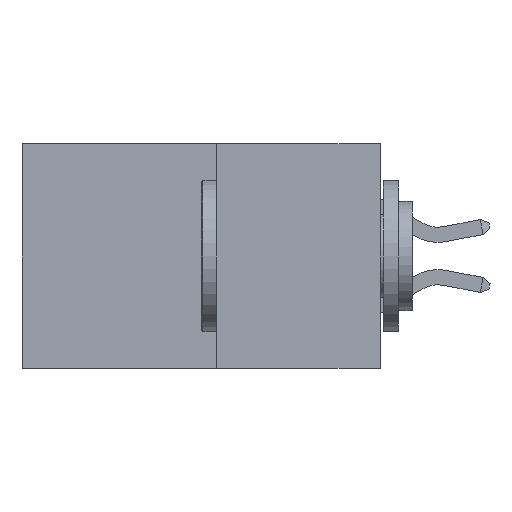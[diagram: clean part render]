
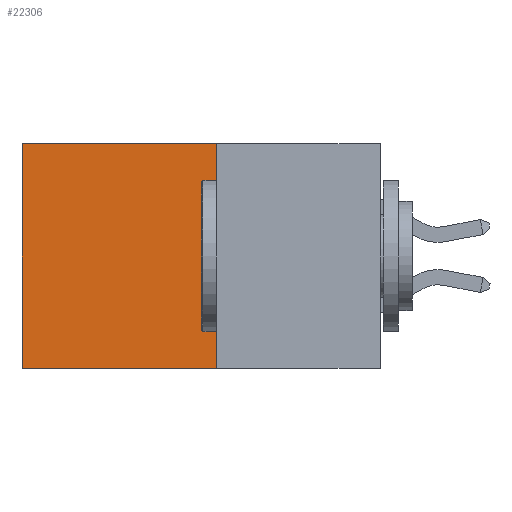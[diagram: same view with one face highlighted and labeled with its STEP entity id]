
A CAD part, left-side view. The second image highlights one B-rep face of the part: STEP entity #22306.
In plain terms, the highlighted planar face has unit normal (-1, 0, 0).
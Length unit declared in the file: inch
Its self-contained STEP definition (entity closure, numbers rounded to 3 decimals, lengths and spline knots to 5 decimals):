
#180 = ORIENTED_EDGE ( 'NONE', *, *, #5512, .T. ) ;
#1679 = AXIS2_PLACEMENT_3D ( 'NONE', #9399, #27180, #11938 ) ;
#3435 = CARTESIAN_POINT ( 'NONE',  ( 0.277, 0.27, 0. ) ) ;
#4235 = PLANE ( 'NONE',  #1679 ) ;
#5512 = EDGE_CURVE ( 'NONE', #9142, #13987, #30243, .T. ) ;
#5621 = EDGE_CURVE ( 'NONE', #30996, #9142, #13556, .T. ) ;
#6481 = CARTESIAN_POINT ( 'NONE',  ( 0.277, 0.59, -0.37 ) ) ;
#7763 = DIRECTION ( 'NONE',  ( 0., 0., -1. ) ) ;
#8308 = DIRECTION ( 'NONE',  ( 0., 1., 0. ) ) ;
#9009 = VECTOR ( 'NONE', #21920, 39.37008 ) ;
#9142 = VERTEX_POINT ( 'NONE', #32840 ) ;
#9253 = FACE_OUTER_BOUND ( 'NONE', #22468, .T. ) ;
#9399 = CARTESIAN_POINT ( 'NONE',  ( 0.277, 0.27, -0.37 ) ) ;
#11687 = CARTESIAN_POINT ( 'NONE',  ( 0.277, 0.27, -0.37 ) ) ;
#11938 = DIRECTION ( 'NONE',  ( 0., 0., -1. ) ) ;
#12021 = VERTEX_POINT ( 'NONE', #28474 ) ;
#12322 = EDGE_CURVE ( 'NONE', #12021, #13987, #23299, .T. ) ;
#13023 = ORIENTED_EDGE ( 'NONE', *, *, #12322, .F. ) ;
#13556 = LINE ( 'NONE', #21056, #19502 ) ;
#13987 = VERTEX_POINT ( 'NONE', #29155 ) ;
#14317 = ORIENTED_EDGE ( 'NONE', *, *, #27354, .F. ) ;
#17378 = VECTOR ( 'NONE', #19501, 39.37008 ) ;
#17708 = ORIENTED_EDGE ( 'NONE', *, *, #5621, .T. ) ;
#19501 = DIRECTION ( 'NONE',  ( 0., 0., -1. ) ) ;
#19502 = VECTOR ( 'NONE', #8308, 39.37008 ) ;
#21056 = CARTESIAN_POINT ( 'NONE',  ( 0.277, 0.27, 0. ) ) ;
#21920 = DIRECTION ( 'NONE',  ( 0., 1., 0. ) ) ;
#22306 = ADVANCED_FACE ( 'NONE', ( #9253 ), #4235, .F. ) ;
#22468 = EDGE_LOOP ( 'NONE', ( #180, #13023, #14317, #17708 ) ) ;
#23299 = LINE ( 'NONE', #11687, #9009 ) ;
#23492 = VECTOR ( 'NONE', #7763, 39.37008 ) ;
#27180 = DIRECTION ( 'NONE',  ( 1., 0., 0. ) ) ;
#27354 = EDGE_CURVE ( 'NONE', #30996, #12021, #31601, .T. ) ;
#28474 = CARTESIAN_POINT ( 'NONE',  ( 0.277, 0.27, -0.37 ) ) ;
#29155 = CARTESIAN_POINT ( 'NONE',  ( 0.277, 0.59, -0.37 ) ) ;
#29611 = CARTESIAN_POINT ( 'NONE',  ( 0.277, 0.27, -0.37 ) ) ;
#30243 = LINE ( 'NONE', #6481, #23492 ) ;
#30996 = VERTEX_POINT ( 'NONE', #3435 ) ;
#31601 = LINE ( 'NONE', #29611, #17378 ) ;
#32840 = CARTESIAN_POINT ( 'NONE',  ( 0.277, 0.59, 0. ) ) ;
